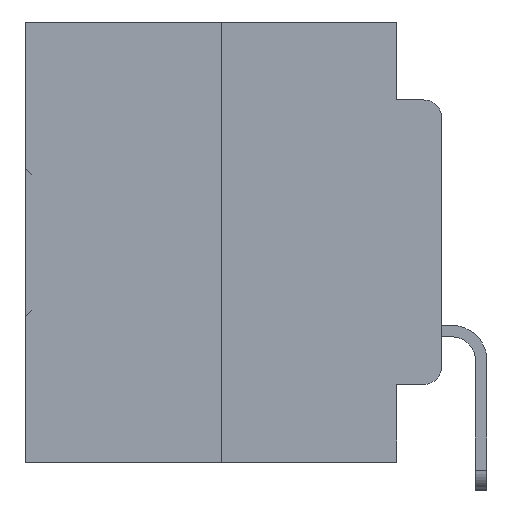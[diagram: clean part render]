
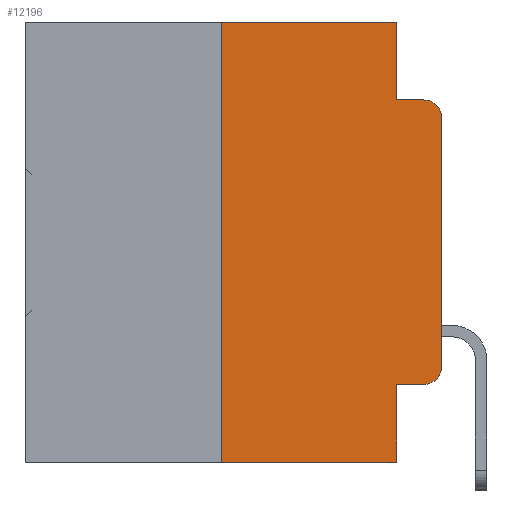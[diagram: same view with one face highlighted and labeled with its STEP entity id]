
A CAD part, left-side view. The second image highlights one B-rep face of the part: STEP entity #12196.
In plain terms, the highlighted planar face has unit normal (-1, 0, 0).
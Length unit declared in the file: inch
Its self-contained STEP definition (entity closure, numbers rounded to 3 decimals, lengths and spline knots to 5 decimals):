
#591 = DIRECTION ( 'NONE',  ( -1., 0., 0. ) ) ;
#1884 = CARTESIAN_POINT ( 'NONE',  ( 0., 0.051, -0.5 ) ) ;
#2380 = LINE ( 'NONE', #18721, #28772 ) ;
#2515 = CARTESIAN_POINT ( 'NONE',  ( 0., 0.473, 0. ) ) ;
#2581 = EDGE_CURVE ( 'NONE', #31243, #27325, #27353, .T. ) ;
#2595 = CARTESIAN_POINT ( 'NONE',  ( 0., 0.02, -0.0885 ) ) ;
#2624 = DIRECTION ( 'NONE',  ( 0., -1., 0. ) ) ;
#2882 = CARTESIAN_POINT ( 'NONE',  ( 0., 0.473, 0. ) ) ;
#3045 = VECTOR ( 'NONE', #25677, 39.37008 ) ;
#3767 = CARTESIAN_POINT ( 'NONE',  ( 0., 0.051, -0.4115 ) ) ;
#4243 = LINE ( 'NONE', #2515, #24388 ) ;
#5104 = ORIENTED_EDGE ( 'NONE', *, *, #10723, .F. ) ;
#5413 = DIRECTION ( 'NONE',  ( 0., -1., 0. ) ) ;
#5762 = DIRECTION ( 'NONE',  ( 0., 0., -1. ) ) ;
#6313 = CARTESIAN_POINT ( 'NONE',  ( 0., 0.051, 0. ) ) ;
#6393 = EDGE_CURVE ( 'NONE', #22784, #31243, #24135, .T. ) ;
#6463 = VECTOR ( 'NONE', #30342, 39.37008 ) ;
#6528 = LINE ( 'NONE', #6916, #21323 ) ;
#6883 = ORIENTED_EDGE ( 'NONE', *, *, #8344, .F. ) ;
#6916 = CARTESIAN_POINT ( 'NONE',  ( 0., 0.25, 0. ) ) ;
#7110 = EDGE_CURVE ( 'NONE', #23935, #22784, #33572, .T. ) ;
#7455 = AXIS2_PLACEMENT_3D ( 'NONE', #16954, #591, #19554 ) ;
#8078 = EDGE_CURVE ( 'NONE', #24604, #21955, #14326, .T. ) ;
#8344 = EDGE_CURVE ( 'NONE', #12153, #21666, #4243, .T. ) ;
#8357 = CARTESIAN_POINT ( 'NONE',  ( 0., 0.25, 0. ) ) ;
#8637 = ORIENTED_EDGE ( 'NONE', *, *, #26239, .F. ) ;
#8935 = EDGE_CURVE ( 'NONE', #15554, #23935, #2380, .T. ) ;
#9166 = CARTESIAN_POINT ( 'NONE',  ( 0., 0.051, -0.0885 ) ) ;
#9463 = AXIS2_PLACEMENT_3D ( 'NONE', #2882, #21513, #5762 ) ;
#10723 = EDGE_CURVE ( 'NONE', #15554, #21955, #11551, .T. ) ;
#10759 = DIRECTION ( 'NONE',  ( 0., -1., 0. ) ) ;
#11102 = PLANE ( 'NONE',  #9463 ) ;
#11551 = LINE ( 'NONE', #6313, #16841 ) ;
#11687 = CARTESIAN_POINT ( 'NONE',  ( 0., 0.051, 0. ) ) ;
#11782 = CARTESIAN_POINT ( 'NONE',  ( 0., 0.02, -0.3915 ) ) ;
#12153 = VERTEX_POINT ( 'NONE', #8357 ) ;
#12196 = ADVANCED_FACE ( 'NONE', ( #31140 ), #11102, .F. ) ;
#13908 = ORIENTED_EDGE ( 'NONE', *, *, #24531, .F. ) ;
#14326 = LINE ( 'NONE', #17512, #6463 ) ;
#14363 = DIRECTION ( 'NONE',  ( 0., 0., -1. ) ) ;
#14496 = LINE ( 'NONE', #28750, #21411 ) ;
#14888 = DIRECTION ( 'NONE',  ( 0., 0., 1. ) ) ;
#15399 = CARTESIAN_POINT ( 'NONE',  ( 0., 0., -0.1085 ) ) ;
#15554 = VERTEX_POINT ( 'NONE', #3767 ) ;
#15957 = ORIENTED_EDGE ( 'NONE', *, *, #8078, .T. ) ;
#16841 = VECTOR ( 'NONE', #16976, 39.37008 ) ;
#16954 = CARTESIAN_POINT ( 'NONE',  ( 0., 0.02, -0.1085 ) ) ;
#16976 = DIRECTION ( 'NONE',  ( 0., 0., -1. ) ) ;
#17512 = CARTESIAN_POINT ( 'NONE',  ( 0., 0.473, -0.5 ) ) ;
#18721 = CARTESIAN_POINT ( 'NONE',  ( 0., 0.051, -0.4115 ) ) ;
#18765 = CARTESIAN_POINT ( 'NONE',  ( 0., 0., -0.3915 ) ) ;
#19554 = DIRECTION ( 'NONE',  ( 0., 0., -1. ) ) ;
#19873 = CARTESIAN_POINT ( 'NONE',  ( 0., 0.051, 0. ) ) ;
#21143 = EDGE_CURVE ( 'NONE', #24604, #12153, #6528, .T. ) ;
#21323 = VECTOR ( 'NONE', #14888, 39.37008 ) ;
#21411 = VECTOR ( 'NONE', #10759, 39.37008 ) ;
#21513 = DIRECTION ( 'NONE',  ( 1., 0., 0. ) ) ;
#21666 = VERTEX_POINT ( 'NONE', #11687 ) ;
#21955 = VERTEX_POINT ( 'NONE', #1884 ) ;
#22361 = ORIENTED_EDGE ( 'NONE', *, *, #8935, .T. ) ;
#22784 = VERTEX_POINT ( 'NONE', #18765 ) ;
#23029 = VERTEX_POINT ( 'NONE', #9166 ) ;
#23874 = AXIS2_PLACEMENT_3D ( 'NONE', #11782, #29756, #14363 ) ;
#23935 = VERTEX_POINT ( 'NONE', #29887 ) ;
#24135 = LINE ( 'NONE', #28279, #3045 ) ;
#24388 = VECTOR ( 'NONE', #5413, 39.37008 ) ;
#24531 = EDGE_CURVE ( 'NONE', #21666, #23029, #27913, .T. ) ;
#24604 = VERTEX_POINT ( 'NONE', #32819 ) ;
#24949 = DIRECTION ( 'NONE',  ( 0., 0., -1. ) ) ;
#25240 = EDGE_LOOP ( 'NONE', ( #25614, #30002, #8637, #13908, #6883, #31175, #15957, #5104, #22361, #31147 ) ) ;
#25614 = ORIENTED_EDGE ( 'NONE', *, *, #6393, .T. ) ;
#25677 = DIRECTION ( 'NONE',  ( 0., 0., 1. ) ) ;
#26239 = EDGE_CURVE ( 'NONE', #23029, #27325, #14496, .T. ) ;
#27325 = VERTEX_POINT ( 'NONE', #2595 ) ;
#27353 = CIRCLE ( 'NONE', #7455, 0.02 ) ;
#27913 = LINE ( 'NONE', #19873, #33027 ) ;
#28279 = CARTESIAN_POINT ( 'NONE',  ( 0., 0., 0. ) ) ;
#28750 = CARTESIAN_POINT ( 'NONE',  ( 0., 0.051, -0.0885 ) ) ;
#28772 = VECTOR ( 'NONE', #2624, 39.37008 ) ;
#29756 = DIRECTION ( 'NONE',  ( -1., 0., 0. ) ) ;
#29887 = CARTESIAN_POINT ( 'NONE',  ( 0., 0.02, -0.4115 ) ) ;
#30002 = ORIENTED_EDGE ( 'NONE', *, *, #2581, .T. ) ;
#30342 = DIRECTION ( 'NONE',  ( 0., -1., 0. ) ) ;
#31140 = FACE_OUTER_BOUND ( 'NONE', #25240, .T. ) ;
#31147 = ORIENTED_EDGE ( 'NONE', *, *, #7110, .T. ) ;
#31175 = ORIENTED_EDGE ( 'NONE', *, *, #21143, .F. ) ;
#31243 = VERTEX_POINT ( 'NONE', #15399 ) ;
#32819 = CARTESIAN_POINT ( 'NONE',  ( 0., 0.25, -0.5 ) ) ;
#33027 = VECTOR ( 'NONE', #24949, 39.37008 ) ;
#33572 = CIRCLE ( 'NONE', #23874, 0.02 ) ;
